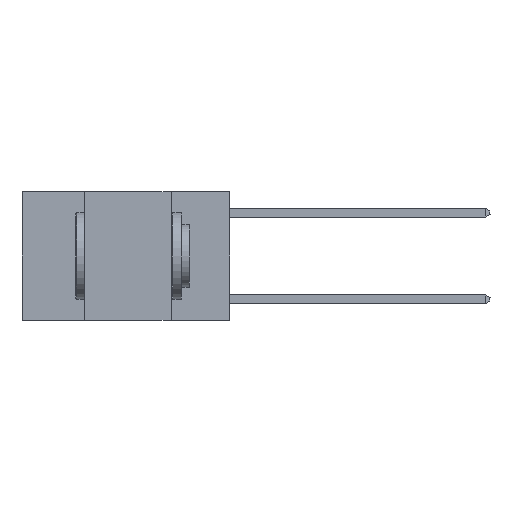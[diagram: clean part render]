
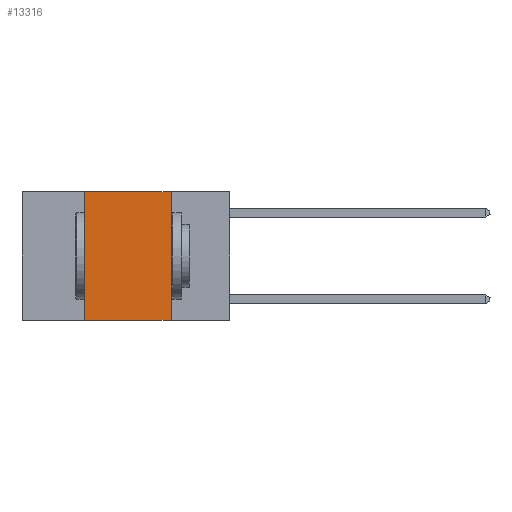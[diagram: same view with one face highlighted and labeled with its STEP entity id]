
A CAD part, left-side view. The second image highlights one B-rep face of the part: STEP entity #13316.
In plain terms, the highlighted planar face has unit normal (-1, 0, 0).
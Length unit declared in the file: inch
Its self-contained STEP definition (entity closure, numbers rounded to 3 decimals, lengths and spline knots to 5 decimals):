
#145 = ORIENTED_EDGE ( 'NONE', *, *, #8602, .F. ) ;
#415 = LINE ( 'NONE', #11610, #12376 ) ;
#801 = EDGE_CURVE ( 'NONE', #9016, #4067, #415, .T. ) ;
#835 = CARTESIAN_POINT ( 'NONE',  ( 0., 0.42, 0. ) ) ;
#1397 = ORIENTED_EDGE ( 'NONE', *, *, #5918, .F. ) ;
#1785 = VECTOR ( 'NONE', #8128, 39.37008 ) ;
#1903 = VERTEX_POINT ( 'NONE', #9043 ) ;
#4067 = VERTEX_POINT ( 'NONE', #10192 ) ;
#4231 = DIRECTION ( 'NONE',  ( 0., -1., 0. ) ) ;
#4343 = LINE ( 'NONE', #9348, #1785 ) ;
#5620 = EDGE_CURVE ( 'NONE', #1903, #4067, #8966, .T. ) ;
#5918 = EDGE_CURVE ( 'NONE', #9016, #12724, #4343, .T. ) ;
#6276 = DIRECTION ( 'NONE',  ( 0., 0., -1. ) ) ;
#6286 = VECTOR ( 'NONE', #6276, 39.37008 ) ;
#6506 = CARTESIAN_POINT ( 'NONE',  ( 0., 0.17, 0. ) ) ;
#6673 = AXIS2_PLACEMENT_3D ( 'NONE', #9689, #14698, #15601 ) ;
#7745 = LINE ( 'NONE', #12748, #10394 ) ;
#8128 = DIRECTION ( 'NONE',  ( 0., 0., 1. ) ) ;
#8560 = FACE_OUTER_BOUND ( 'NONE', #14932, .T. ) ;
#8602 = EDGE_CURVE ( 'NONE', #12724, #1903, #7745, .T. ) ;
#8966 = LINE ( 'NONE', #6506, #6286 ) ;
#9016 = VERTEX_POINT ( 'NONE', #12337 ) ;
#9043 = CARTESIAN_POINT ( 'NONE',  ( 0., 0.17, 0. ) ) ;
#9348 = CARTESIAN_POINT ( 'NONE',  ( 0., 0.42, 0. ) ) ;
#9689 = CARTESIAN_POINT ( 'NONE',  ( 0., 0.6, 0. ) ) ;
#10192 = CARTESIAN_POINT ( 'NONE',  ( 0., 0.17, -0.37 ) ) ;
#10394 = VECTOR ( 'NONE', #14131, 39.37008 ) ;
#10670 = ORIENTED_EDGE ( 'NONE', *, *, #5620, .F. ) ;
#11610 = CARTESIAN_POINT ( 'NONE',  ( 0., 0.6, -0.37 ) ) ;
#12003 = PLANE ( 'NONE',  #6673 ) ;
#12337 = CARTESIAN_POINT ( 'NONE',  ( 0., 0.42, -0.37 ) ) ;
#12376 = VECTOR ( 'NONE', #4231, 39.37008 ) ;
#12724 = VERTEX_POINT ( 'NONE', #835 ) ;
#12748 = CARTESIAN_POINT ( 'NONE',  ( 0., 0.6, 0. ) ) ;
#13316 = ADVANCED_FACE ( 'NONE', ( #8560 ), #12003, .F. ) ;
#13578 = ORIENTED_EDGE ( 'NONE', *, *, #801, .T. ) ;
#14131 = DIRECTION ( 'NONE',  ( 0., -1., 0. ) ) ;
#14698 = DIRECTION ( 'NONE',  ( 1., 0., 0. ) ) ;
#14932 = EDGE_LOOP ( 'NONE', ( #10670, #145, #1397, #13578 ) ) ;
#15601 = DIRECTION ( 'NONE',  ( 0., 0., -1. ) ) ;
